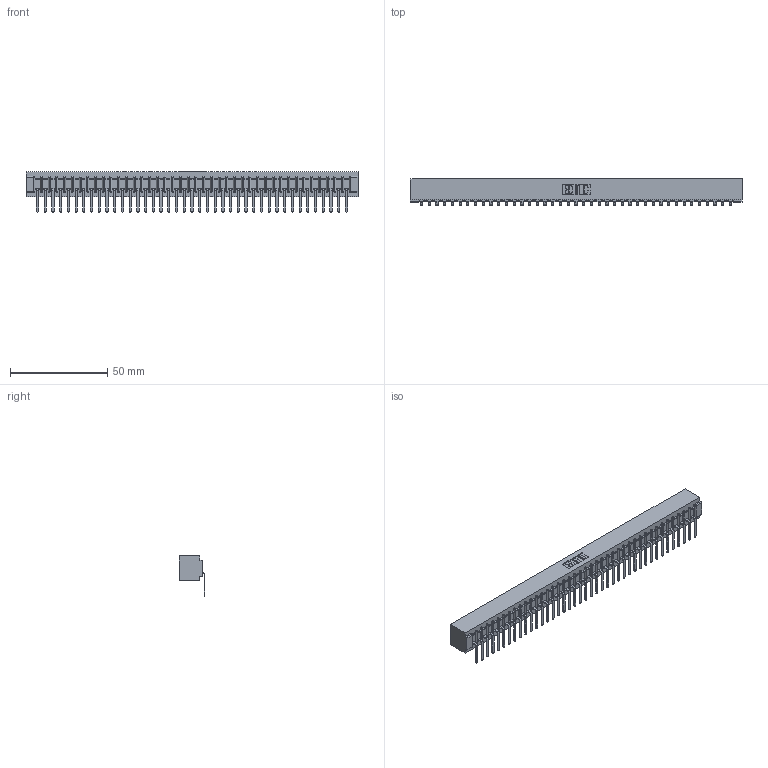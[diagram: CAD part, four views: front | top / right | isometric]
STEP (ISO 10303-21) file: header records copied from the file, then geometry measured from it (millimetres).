
FILE_DESCRIPTION (( 'STEP AP203' ), '1' );
FILE_NAME ('357-041-457-101.STEP', '2020-10-03T08:59:50', ( '' ), ( '' ), 'SwSTEP 2.0', 'SolidWorks 2020', '' );
FILE_SCHEMA (( 'CONFIG_CONTROL_DESIGN' ));
Length unit declared in the file: inch
Products named in the file (3): 307 Part_No Mounting Lugs; 357-041-457-101; 307-290-002_557
Assembly tree (42 placements, depth 2):
  357-041-457-101
    307 Part_No Mounting Lugs
    307-290-002_557  x41
Bounding box: 170.33 x 13.32 x 20.66 mm (x, y, z)
Volume: 18888.7 mm3; surface area: 24796.6 mm2
Topology: 42 solids, 42 shells, 3350 faces, 10303 edges, 6754 vertices
Faces by surface type: plane 1993, cylinder 1273, sphere 84
Entity records: 35848 total; most frequent: CARTESIAN_POINT 6048, ORIENTED_EDGE 6038, DIRECTION 5875, EDGE_CURVE 3019, VECTOR 2313, LINE 2313, VERTEX_POINT 1954, AXIS2_PLACEMENT_3D 1781
